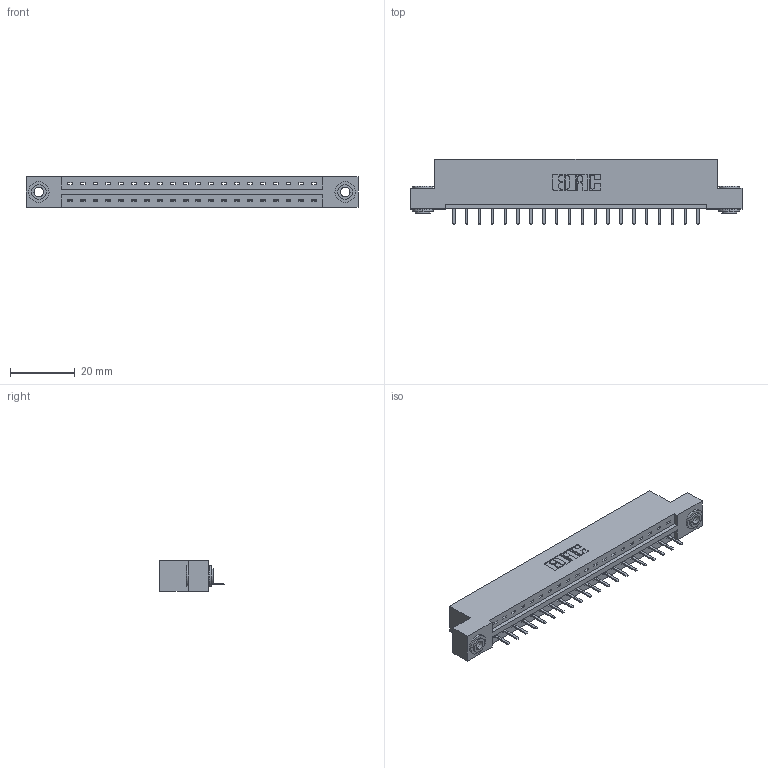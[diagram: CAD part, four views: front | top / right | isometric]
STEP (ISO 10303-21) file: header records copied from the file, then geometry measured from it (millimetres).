
FILE_DESCRIPTION (( 'STEP AP203' ), '1' );
FILE_NAME ('387-020-520-103.STEP', '2018-09-13T06:26:48', ( '' ), ( '' ), 'SwSTEP 2.0', 'SolidWorks 2016', '' );
FILE_SCHEMA (( 'CONFIG_CONTROL_DESIGN' ));
Length unit declared in the file: inch
Products named in the file (4): 345-250-002_345-250-002-102; 387-020-520-103; 337 Part_Flush Mounting Lugs - 0.156 Dia-TH; 345-292-001_345-293-120
Assembly tree (23 placements, depth 2):
  387-020-520-103
    337 Part_Flush Mounting Lugs - 0.156 Dia-TH
    345-292-001_345-293-120  x20
    345-250-002_345-250-002-102  x2
Bounding box: 102.26 x 20.02 x 9.4 mm (x, y, z)
Volume: 10314.8 mm3; surface area: 10562.4 mm2
Topology: 23 solids, 23 shells, 1472 faces, 4307 edges, 2814 vertices
Faces by surface type: plane 1040, cylinder 424, cone 8
Entity records: 18476 total; most frequent: CARTESIAN_POINT 3205, ORIENTED_EDGE 3142, DIRECTION 2765, EDGE_CURVE 1571, VECTOR 1415, LINE 1415, VERTEX_POINT 1042, AXIS2_PLACEMENT_3D 675
